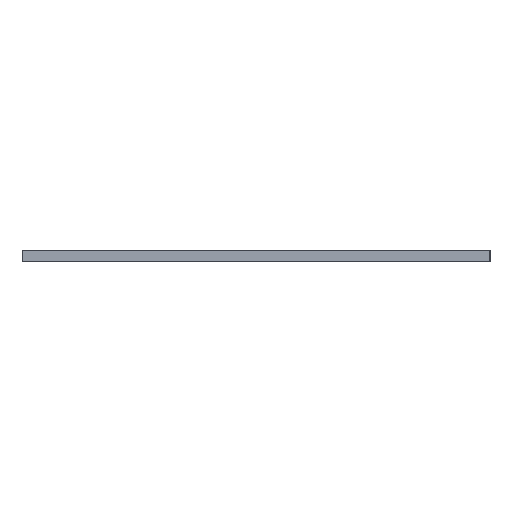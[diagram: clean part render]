
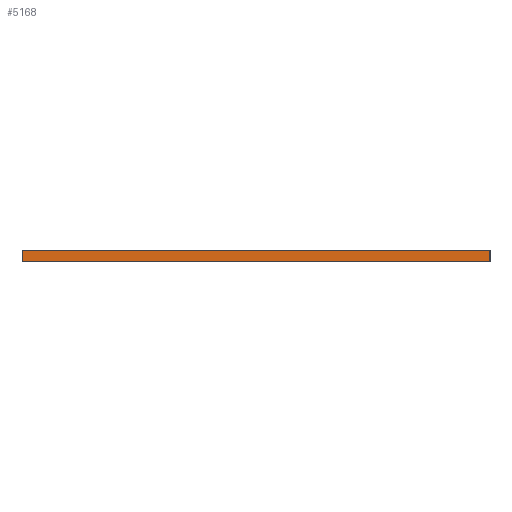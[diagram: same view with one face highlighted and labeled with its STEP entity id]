
A CAD part, front view. The second image highlights one B-rep face of the part: STEP entity #5168.
In plain terms, the highlighted planar face has unit normal (0, -1, 0).
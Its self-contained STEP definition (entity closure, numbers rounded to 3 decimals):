
#92 = ORIENTED_EDGE ( 'NONE', *, *, #1729, .T. ) ;
#706 = DIRECTION ( 'NONE',  ( -1., 0., 0. ) ) ;
#813 = PLANE ( 'NONE',  #3686 ) ;
#1173 = EDGE_CURVE ( 'NONE', #4523, #6258, #10129, .T. ) ;
#1241 = CARTESIAN_POINT ( 'NONE',  ( -22.811, -19.5, 21.127 ) ) ;
#1729 = EDGE_CURVE ( 'NONE', #15080, #3045, #16606, .T. ) ;
#1735 = CARTESIAN_POINT ( 'NONE',  ( 17.189, -19.5, 22.127 ) ) ;
#2176 = DIRECTION ( 'NONE',  ( 1., 0., 0. ) ) ;
#2418 = VECTOR ( 'NONE', #12147, 1000. ) ;
#3045 = VERTEX_POINT ( 'NONE', #9585 ) ;
#3686 = AXIS2_PLACEMENT_3D ( 'NONE', #8903, #10215, #2176 ) ;
#3853 = EDGE_CURVE ( 'NONE', #6258, #3045, #5892, .T. ) ;
#4523 = VERTEX_POINT ( 'NONE', #14035 ) ;
#4778 = CARTESIAN_POINT ( 'NONE',  ( 17.189, -19.5, 21.127 ) ) ;
#4959 = EDGE_LOOP ( 'NONE', ( #92, #5620, #16414, #5922 ) ) ;
#5168 = ADVANCED_FACE ( 'NONE', ( #12224 ), #813, .F. ) ;
#5549 = CARTESIAN_POINT ( 'NONE',  ( -22.811, -19.5, 21.127 ) ) ;
#5620 = ORIENTED_EDGE ( 'NONE', *, *, #3853, .F. ) ;
#5892 = LINE ( 'NONE', #7573, #12445 ) ;
#5922 = ORIENTED_EDGE ( 'NONE', *, *, #13863, .T. ) ;
#6258 = VERTEX_POINT ( 'NONE', #5549 ) ;
#6294 = VECTOR ( 'NONE', #13905, 1000. ) ;
#7573 = CARTESIAN_POINT ( 'NONE',  ( -22.811, -19.5, 21.127 ) ) ;
#8051 = DIRECTION ( 'NONE',  ( 0., 0., 1. ) ) ;
#8903 = CARTESIAN_POINT ( 'NONE',  ( -22.811, -19.5, 21.127 ) ) ;
#9585 = CARTESIAN_POINT ( 'NONE',  ( -22.811, -19.5, 22.127 ) ) ;
#10129 = LINE ( 'NONE', #1241, #13098 ) ;
#10215 = DIRECTION ( 'NONE',  ( 0., 1., 0. ) ) ;
#11812 = CARTESIAN_POINT ( 'NONE',  ( -22.811, -19.5, 22.127 ) ) ;
#12147 = DIRECTION ( 'NONE',  ( -1., 0., 0. ) ) ;
#12224 = FACE_OUTER_BOUND ( 'NONE', #4959, .T. ) ;
#12445 = VECTOR ( 'NONE', #8051, 1000. ) ;
#13098 = VECTOR ( 'NONE', #706, 1000. ) ;
#13863 = EDGE_CURVE ( 'NONE', #4523, #15080, #16471, .T. ) ;
#13905 = DIRECTION ( 'NONE',  ( 0., 0., 1. ) ) ;
#14035 = CARTESIAN_POINT ( 'NONE',  ( 17.189, -19.5, 21.127 ) ) ;
#15080 = VERTEX_POINT ( 'NONE', #1735 ) ;
#16414 = ORIENTED_EDGE ( 'NONE', *, *, #1173, .F. ) ;
#16471 = LINE ( 'NONE', #4778, #6294 ) ;
#16606 = LINE ( 'NONE', #11812, #2418 ) ;
